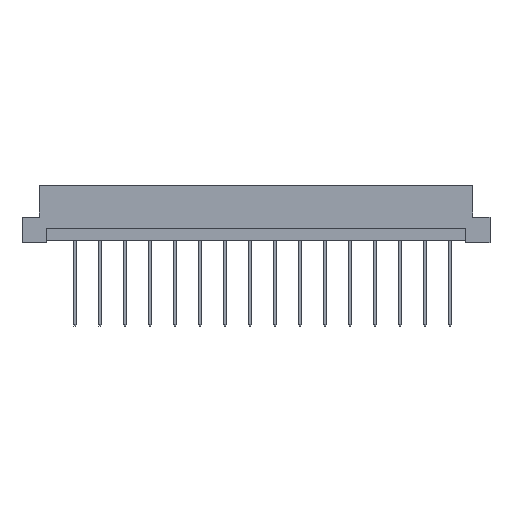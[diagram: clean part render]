
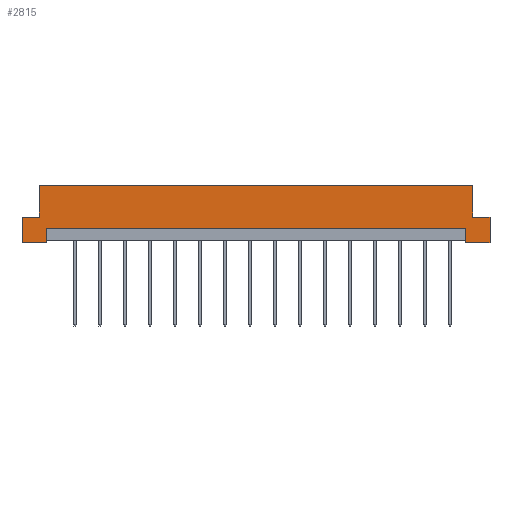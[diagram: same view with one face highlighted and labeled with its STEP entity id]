
A CAD part, front view. The second image highlights one B-rep face of the part: STEP entity #2815.
In plain terms, the highlighted planar face has unit normal (0, -1, 0).
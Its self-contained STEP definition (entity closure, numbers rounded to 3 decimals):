
#99 = ORIENTED_EDGE ( 'NONE', *, *, #7317, .T. ) ;
#221 = VECTOR ( 'NONE', #15042, 1000. ) ;
#293 = ORIENTED_EDGE ( 'NONE', *, *, #8467, .F. ) ;
#304 = VECTOR ( 'NONE', #9637, 1000. ) ;
#360 = CARTESIAN_POINT ( 'NONE',  ( 47.5, 0., 5.2 ) ) ;
#617 = DIRECTION ( 'NONE',  ( -1., 0., 0. ) ) ;
#801 = DIRECTION ( 'NONE',  ( 1., 0., 0. ) ) ;
#822 = CARTESIAN_POINT ( 'NONE',  ( -44., 0., 5.2 ) ) ;
#942 = ORIENTED_EDGE ( 'NONE', *, *, #13532, .F. ) ;
#951 = EDGE_CURVE ( 'NONE', #2601, #2162, #11772, .T. ) ;
#1117 = EDGE_CURVE ( 'NONE', #14134, #11067, #7196, .T. ) ;
#1177 = EDGE_LOOP ( 'NONE', ( #5701, #11644, #9135, #942, #7699, #99, #293, #9602, #6334, #15528, #5403, #13443 ) ) ;
#1234 = CARTESIAN_POINT ( 'NONE',  ( -44., 0., 11.6 ) ) ;
#1315 = EDGE_CURVE ( 'NONE', #6004, #5651, #12489, .T. ) ;
#1333 = VERTEX_POINT ( 'NONE', #7680 ) ;
#1619 = DIRECTION ( 'NONE',  ( -1., 0., 0. ) ) ;
#1663 = LINE ( 'NONE', #12717, #221 ) ;
#1674 = DIRECTION ( 'NONE',  ( 0., 0., 1. ) ) ;
#1730 = VECTOR ( 'NONE', #10055, 1000. ) ;
#1888 = EDGE_CURVE ( 'NONE', #12806, #13318, #12950, .T. ) ;
#2071 = VECTOR ( 'NONE', #12677, 1000. ) ;
#2162 = VERTEX_POINT ( 'NONE', #360 ) ;
#2278 = VECTOR ( 'NONE', #5958, 1000. ) ;
#2601 = VERTEX_POINT ( 'NONE', #10028 ) ;
#2815 = ADVANCED_FACE ( 'NONE', ( #8179 ), #5909, .F. ) ;
#2839 = LINE ( 'NONE', #13895, #1730 ) ;
#3194 = VERTEX_POINT ( 'NONE', #4530 ) ;
#3330 = EDGE_CURVE ( 'NONE', #1333, #13318, #9586, .T. ) ;
#3635 = CARTESIAN_POINT ( 'NONE',  ( 42.6, 0., 0.5 ) ) ;
#3739 = DIRECTION ( 'NONE',  ( 0., 1., 0. ) ) ;
#4530 = CARTESIAN_POINT ( 'NONE',  ( 44., 0., 11.6 ) ) ;
#4636 = CARTESIAN_POINT ( 'NONE',  ( -47.5, 0., 11.6 ) ) ;
#4717 = CARTESIAN_POINT ( 'NONE',  ( -47.5, 0., 0. ) ) ;
#4944 = LINE ( 'NONE', #9845, #12504 ) ;
#5403 = ORIENTED_EDGE ( 'NONE', *, *, #8999, .F. ) ;
#5651 = VERTEX_POINT ( 'NONE', #1234 ) ;
#5686 = DIRECTION ( 'NONE',  ( 0., 0., 1. ) ) ;
#5701 = ORIENTED_EDGE ( 'NONE', *, *, #9452, .F. ) ;
#5909 = PLANE ( 'NONE',  #9028 ) ;
#5937 = CARTESIAN_POINT ( 'NONE',  ( -42.6, 0., 0.5 ) ) ;
#5958 = DIRECTION ( 'NONE',  ( 0., 0., -1. ) ) ;
#6004 = VERTEX_POINT ( 'NONE', #822 ) ;
#6334 = ORIENTED_EDGE ( 'NONE', *, *, #8480, .F. ) ;
#6777 = VECTOR ( 'NONE', #12002, 1000. ) ;
#7196 = LINE ( 'NONE', #4717, #6777 ) ;
#7317 = EDGE_CURVE ( 'NONE', #2601, #3194, #13869, .T. ) ;
#7367 = LINE ( 'NONE', #14583, #13337 ) ;
#7428 = DIRECTION ( 'NONE',  ( 1., 0., 0. ) ) ;
#7552 = CARTESIAN_POINT ( 'NONE',  ( 42.6, 0., 2.9 ) ) ;
#7680 = CARTESIAN_POINT ( 'NONE',  ( 42.6, 0., 2.9 ) ) ;
#7699 = ORIENTED_EDGE ( 'NONE', *, *, #951, .F. ) ;
#8179 = FACE_OUTER_BOUND ( 'NONE', #1177, .T. ) ;
#8467 = EDGE_CURVE ( 'NONE', #5651, #3194, #4944, .T. ) ;
#8480 = EDGE_CURVE ( 'NONE', #11067, #6004, #1663, .T. ) ;
#8999 = EDGE_CURVE ( 'NONE', #12127, #14134, #2839, .T. ) ;
#9024 = CARTESIAN_POINT ( 'NONE',  ( -47.5, 0., 0. ) ) ;
#9028 = AXIS2_PLACEMENT_3D ( 'NONE', #4636, #3739, #5686 ) ;
#9135 = ORIENTED_EDGE ( 'NONE', *, *, #1888, .F. ) ;
#9173 = CARTESIAN_POINT ( 'NONE',  ( -42.6, 0., 2.9 ) ) ;
#9452 = EDGE_CURVE ( 'NONE', #1333, #10200, #12755, .T. ) ;
#9586 = LINE ( 'NONE', #3635, #2278 ) ;
#9602 = ORIENTED_EDGE ( 'NONE', *, *, #1315, .F. ) ;
#9637 = DIRECTION ( 'NONE',  ( 0., 0., -1. ) ) ;
#9845 = CARTESIAN_POINT ( 'NONE',  ( -47.5, 0., 11.6 ) ) ;
#10028 = CARTESIAN_POINT ( 'NONE',  ( 44., 0., 5.2 ) ) ;
#10055 = DIRECTION ( 'NONE',  ( -1., 0., 0. ) ) ;
#10200 = VERTEX_POINT ( 'NONE', #9173 ) ;
#10424 = VECTOR ( 'NONE', #1619, 1000. ) ;
#11067 = VERTEX_POINT ( 'NONE', #13933 ) ;
#11622 = CARTESIAN_POINT ( 'NONE',  ( 47.5, 0., 5.2 ) ) ;
#11644 = ORIENTED_EDGE ( 'NONE', *, *, #3330, .T. ) ;
#11772 = LINE ( 'NONE', #11622, #15471 ) ;
#11865 = CARTESIAN_POINT ( 'NONE',  ( -42.6, 0., 0. ) ) ;
#12002 = DIRECTION ( 'NONE',  ( 0., 0., 1. ) ) ;
#12127 = VERTEX_POINT ( 'NONE', #11865 ) ;
#12489 = LINE ( 'NONE', #12656, #14459 ) ;
#12504 = VECTOR ( 'NONE', #7428, 1000. ) ;
#12656 = CARTESIAN_POINT ( 'NONE',  ( -44., 0., 5.2 ) ) ;
#12677 = DIRECTION ( 'NONE',  ( 0., 0., 1. ) ) ;
#12717 = CARTESIAN_POINT ( 'NONE',  ( -47.5, 0., 5.2 ) ) ;
#12751 = CARTESIAN_POINT ( 'NONE',  ( 44., 0., 5.2 ) ) ;
#12755 = LINE ( 'NONE', #7552, #10424 ) ;
#12806 = VERTEX_POINT ( 'NONE', #13660 ) ;
#12950 = LINE ( 'NONE', #9024, #13638 ) ;
#12958 = CARTESIAN_POINT ( 'NONE',  ( -47.5, 0., 0. ) ) ;
#13051 = EDGE_CURVE ( 'NONE', #10200, #12127, #15650, .T. ) ;
#13318 = VERTEX_POINT ( 'NONE', #13636 ) ;
#13337 = VECTOR ( 'NONE', #15625, 1000. ) ;
#13443 = ORIENTED_EDGE ( 'NONE', *, *, #13051, .F. ) ;
#13532 = EDGE_CURVE ( 'NONE', #2162, #12806, #7367, .T. ) ;
#13636 = CARTESIAN_POINT ( 'NONE',  ( 42.6, 0., 0. ) ) ;
#13638 = VECTOR ( 'NONE', #617, 1000. ) ;
#13660 = CARTESIAN_POINT ( 'NONE',  ( 47.5, 0., 0. ) ) ;
#13869 = LINE ( 'NONE', #12751, #2071 ) ;
#13895 = CARTESIAN_POINT ( 'NONE',  ( -47.5, 0., 0. ) ) ;
#13933 = CARTESIAN_POINT ( 'NONE',  ( -47.5, 0., 5.2 ) ) ;
#14134 = VERTEX_POINT ( 'NONE', #12958 ) ;
#14459 = VECTOR ( 'NONE', #1674, 1000. ) ;
#14583 = CARTESIAN_POINT ( 'NONE',  ( 47.5, 0., 0. ) ) ;
#15042 = DIRECTION ( 'NONE',  ( 1., 0., 0. ) ) ;
#15471 = VECTOR ( 'NONE', #801, 1000. ) ;
#15528 = ORIENTED_EDGE ( 'NONE', *, *, #1117, .F. ) ;
#15625 = DIRECTION ( 'NONE',  ( 0., 0., -1. ) ) ;
#15650 = LINE ( 'NONE', #5937, #304 ) ;
